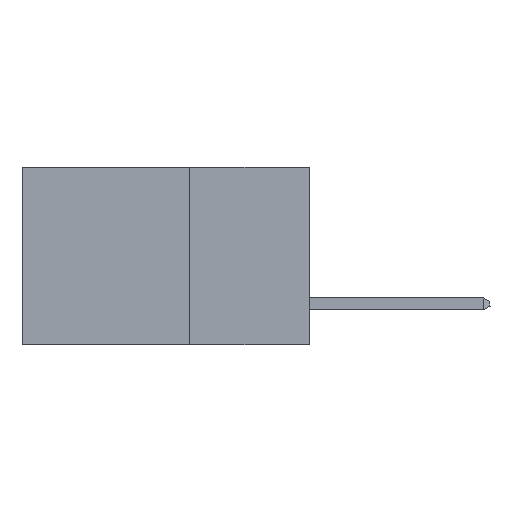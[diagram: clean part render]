
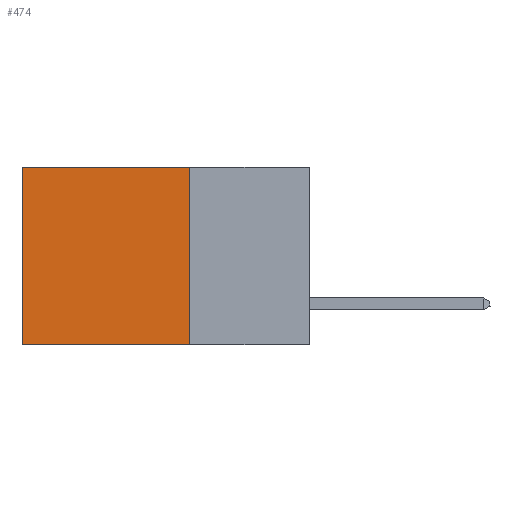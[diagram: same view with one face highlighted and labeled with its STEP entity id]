
A CAD part, left-side view. The second image highlights one B-rep face of the part: STEP entity #474.
In plain terms, the highlighted planar face has unit normal (-1, 0, 0).
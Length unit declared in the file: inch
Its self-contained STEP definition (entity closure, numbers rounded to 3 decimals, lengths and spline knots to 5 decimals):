
#474 = ADVANCED_FACE ( 'NONE', ( #7179 ), #27209, .F. ) ;
#1965 = VERTEX_POINT ( 'NONE', #25193 ) ;
#4518 = ORIENTED_EDGE ( 'NONE', *, *, #14936, .T. ) ;
#5187 = VECTOR ( 'NONE', #25144, 39.37008 ) ;
#5415 = VECTOR ( 'NONE', #12216, 39.37008 ) ;
#6076 = EDGE_CURVE ( 'NONE', #12126, #14183, #12133, .T. ) ;
#7179 = FACE_OUTER_BOUND ( 'NONE', #7500, .T. ) ;
#7500 = EDGE_LOOP ( 'NONE', ( #4518, #20357, #14596, #19279 ) ) ;
#8883 = DIRECTION ( 'NONE',  ( 0., 0., -1. ) ) ;
#9799 = VERTEX_POINT ( 'NONE', #17865 ) ;
#12126 = VERTEX_POINT ( 'NONE', #27296 ) ;
#12133 = LINE ( 'NONE', #21234, #5415 ) ;
#12216 = DIRECTION ( 'NONE',  ( 0., 1., 0. ) ) ;
#13468 = CARTESIAN_POINT ( 'NONE',  ( 0.2875, 0.6, 0. ) ) ;
#14183 = VERTEX_POINT ( 'NONE', #22190 ) ;
#14596 = ORIENTED_EDGE ( 'NONE', *, *, #22743, .F. ) ;
#14936 = EDGE_CURVE ( 'NONE', #14183, #1965, #20981, .T. ) ;
#16254 = CARTESIAN_POINT ( 'NONE',  ( 0.2875, 0.25, -0.37 ) ) ;
#17259 = LINE ( 'NONE', #16254, #5187 ) ;
#17865 = CARTESIAN_POINT ( 'NONE',  ( 0.2875, 0.25, -0.37 ) ) ;
#18108 = EDGE_CURVE ( 'NONE', #9799, #1965, #17259, .T. ) ;
#19279 = ORIENTED_EDGE ( 'NONE', *, *, #6076, .T. ) ;
#20357 = ORIENTED_EDGE ( 'NONE', *, *, #18108, .F. ) ;
#20981 = LINE ( 'NONE', #13468, #26889 ) ;
#21234 = CARTESIAN_POINT ( 'NONE',  ( 0.2875, 0.25, 0. ) ) ;
#22027 = AXIS2_PLACEMENT_3D ( 'NONE', #27432, #27181, #27118 ) ;
#22190 = CARTESIAN_POINT ( 'NONE',  ( 0.2875, 0.6, 0. ) ) ;
#22344 = LINE ( 'NONE', #25992, #28216 ) ;
#22743 = EDGE_CURVE ( 'NONE', #12126, #9799, #22344, .T. ) ;
#25144 = DIRECTION ( 'NONE',  ( 0., 1., 0. ) ) ;
#25193 = CARTESIAN_POINT ( 'NONE',  ( 0.2875, 0.6, -0.37 ) ) ;
#25992 = CARTESIAN_POINT ( 'NONE',  ( 0.2875, 0.25, 0. ) ) ;
#26889 = VECTOR ( 'NONE', #8883, 39.37008 ) ;
#27118 = DIRECTION ( 'NONE',  ( 0., 0., -1. ) ) ;
#27181 = DIRECTION ( 'NONE',  ( 1., 0., 0. ) ) ;
#27209 = PLANE ( 'NONE',  #22027 ) ;
#27296 = CARTESIAN_POINT ( 'NONE',  ( 0.2875, 0.25, 0. ) ) ;
#27432 = CARTESIAN_POINT ( 'NONE',  ( 0.2875, 0.25, 0. ) ) ;
#28192 = DIRECTION ( 'NONE',  ( 0., 0., -1. ) ) ;
#28216 = VECTOR ( 'NONE', #28192, 39.37008 ) ;
